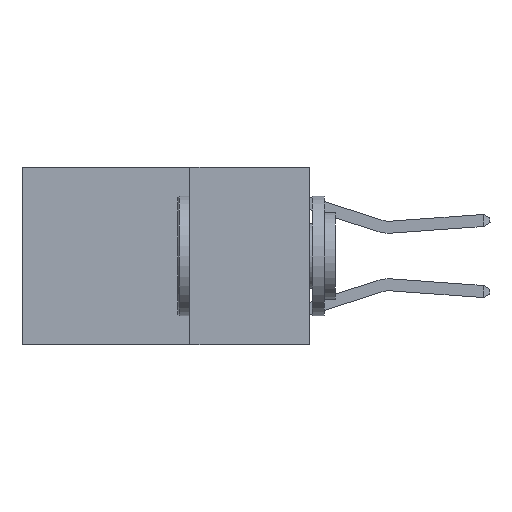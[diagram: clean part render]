
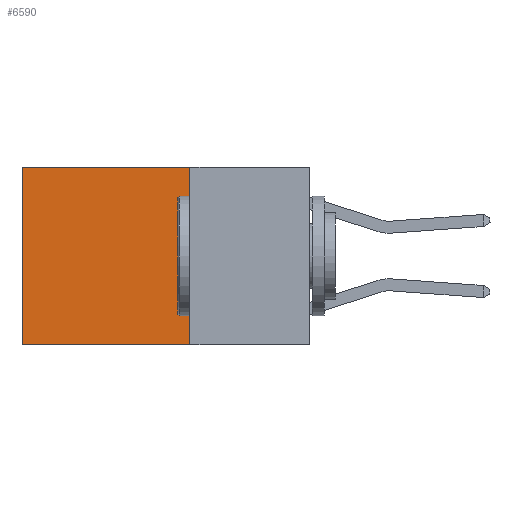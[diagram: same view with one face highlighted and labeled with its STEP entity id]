
A CAD part, left-side view. The second image highlights one B-rep face of the part: STEP entity #6590.
In plain terms, the highlighted planar face has unit normal (-1, 0, 0).
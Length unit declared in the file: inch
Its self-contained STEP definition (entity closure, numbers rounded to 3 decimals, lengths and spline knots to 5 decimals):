
#75 = CARTESIAN_POINT ( 'NONE',  ( 0.2625, 0.6, 0. ) ) ;
#94 = FACE_OUTER_BOUND ( 'NONE', #8791, .T. ) ;
#471 = ORIENTED_EDGE ( 'NONE', *, *, #5472, .F. ) ;
#548 = ORIENTED_EDGE ( 'NONE', *, *, #9462, .T. ) ;
#939 = VERTEX_POINT ( 'NONE', #4265 ) ;
#1091 = PLANE ( 'NONE',  #2494 ) ;
#1236 = DIRECTION ( 'NONE',  ( 0., 0., -1. ) ) ;
#1692 = CARTESIAN_POINT ( 'NONE',  ( 0.2625, 0.25, -0.37 ) ) ;
#1716 = DIRECTION ( 'NONE',  ( 0., 1., 0. ) ) ;
#1945 = DIRECTION ( 'NONE',  ( 1., 0., 0. ) ) ;
#2494 = AXIS2_PLACEMENT_3D ( 'NONE', #6887, #1945, #7686 ) ;
#3055 = CARTESIAN_POINT ( 'NONE',  ( 0.2625, 0.25, 0. ) ) ;
#3452 = CARTESIAN_POINT ( 'NONE',  ( 0.2625, 0.6, -0.37 ) ) ;
#4070 = VECTOR ( 'NONE', #5275, 39.37008 ) ;
#4117 = EDGE_CURVE ( 'NONE', #939, #6540, #9083, .T. ) ;
#4265 = CARTESIAN_POINT ( 'NONE',  ( 0.2625, 0.25, -0.37 ) ) ;
#4362 = LINE ( 'NONE', #6174, #9026 ) ;
#4402 = CARTESIAN_POINT ( 'NONE',  ( 0.2625, 0.25, 0. ) ) ;
#5206 = VECTOR ( 'NONE', #8810, 39.37008 ) ;
#5275 = DIRECTION ( 'NONE',  ( 0., 1., 0. ) ) ;
#5397 = ORIENTED_EDGE ( 'NONE', *, *, #4117, .F. ) ;
#5472 = EDGE_CURVE ( 'NONE', #7715, #939, #7171, .T. ) ;
#6168 = VECTOR ( 'NONE', #1716, 39.37008 ) ;
#6174 = CARTESIAN_POINT ( 'NONE',  ( 0.2625, 0.6, 0. ) ) ;
#6325 = LINE ( 'NONE', #4402, #4070 ) ;
#6523 = ORIENTED_EDGE ( 'NONE', *, *, #7149, .T. ) ;
#6540 = VERTEX_POINT ( 'NONE', #3452 ) ;
#6590 = ADVANCED_FACE ( 'NONE', ( #94 ), #1091, .F. ) ;
#6887 = CARTESIAN_POINT ( 'NONE',  ( 0.2625, 0.25, 0. ) ) ;
#6928 = CARTESIAN_POINT ( 'NONE',  ( 0.2625, 0.25, 0. ) ) ;
#7149 = EDGE_CURVE ( 'NONE', #10408, #6540, #4362, .T. ) ;
#7171 = LINE ( 'NONE', #3055, #5206 ) ;
#7686 = DIRECTION ( 'NONE',  ( 0., 0., -1. ) ) ;
#7715 = VERTEX_POINT ( 'NONE', #6928 ) ;
#8791 = EDGE_LOOP ( 'NONE', ( #6523, #5397, #471, #548 ) ) ;
#8810 = DIRECTION ( 'NONE',  ( 0., 0., -1. ) ) ;
#9026 = VECTOR ( 'NONE', #1236, 39.37008 ) ;
#9083 = LINE ( 'NONE', #1692, #6168 ) ;
#9462 = EDGE_CURVE ( 'NONE', #7715, #10408, #6325, .T. ) ;
#10408 = VERTEX_POINT ( 'NONE', #75 ) ;
